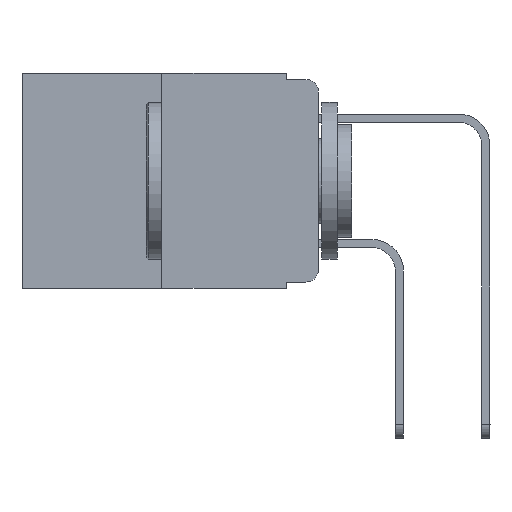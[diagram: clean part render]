
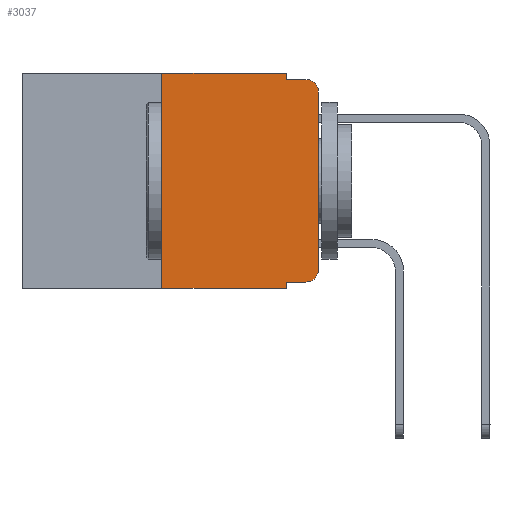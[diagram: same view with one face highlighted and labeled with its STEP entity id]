
A CAD part, left-side view. The second image highlights one B-rep face of the part: STEP entity #3037.
In plain terms, the highlighted planar face has unit normal (-1, 0, 0).
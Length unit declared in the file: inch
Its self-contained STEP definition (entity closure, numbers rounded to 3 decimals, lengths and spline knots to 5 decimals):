
#169 = EDGE_CURVE ( 'NONE', #7126, #14997, #2130, .T. ) ;
#392 = CARTESIAN_POINT ( 'NONE',  ( 0., 0.02, -0.333 ) ) ;
#841 = PLANE ( 'NONE',  #9326 ) ;
#935 = DIRECTION ( 'NONE',  ( 0., 0., -1. ) ) ;
#967 = CARTESIAN_POINT ( 'NONE',  ( 0., 0.051, 0. ) ) ;
#1067 = DIRECTION ( 'NONE',  ( 0., 0., 1. ) ) ;
#1392 = CARTESIAN_POINT ( 'NONE',  ( 0., 0.051, -0.343 ) ) ;
#2130 = LINE ( 'NONE', #6580, #14622 ) ;
#2162 = LINE ( 'NONE', #3811, #18434 ) ;
#2195 = ORIENTED_EDGE ( 'NONE', *, *, #14631, .F. ) ;
#2296 = LINE ( 'NONE', #12321, #9744 ) ;
#2407 = ORIENTED_EDGE ( 'NONE', *, *, #11637, .T. ) ;
#2442 = EDGE_CURVE ( 'NONE', #14997, #15102, #2162, .T. ) ;
#3037 = ADVANCED_FACE ( 'NONE', ( #14137 ), #841, .F. ) ;
#3051 = DIRECTION ( 'NONE',  ( 0., -1., 0. ) ) ;
#3281 = DIRECTION ( 'NONE',  ( 0., -1., 0. ) ) ;
#3811 = CARTESIAN_POINT ( 'NONE',  ( 0., 0.051, -0.01 ) ) ;
#4151 = AXIS2_PLACEMENT_3D ( 'NONE', #17323, #5757, #12860 ) ;
#4877 = DIRECTION ( 'NONE',  ( -1., 0., 0. ) ) ;
#5098 = ORIENTED_EDGE ( 'NONE', *, *, #17485, .T. ) ;
#5145 = CARTESIAN_POINT ( 'NONE',  ( 0., 0.051, -0.333 ) ) ;
#5186 = ORIENTED_EDGE ( 'NONE', *, *, #2442, .F. ) ;
#5389 = ORIENTED_EDGE ( 'NONE', *, *, #169, .F. ) ;
#5433 = CARTESIAN_POINT ( 'NONE',  ( 0., 0.25, 0. ) ) ;
#5496 = LINE ( 'NONE', #18900, #17254 ) ;
#5757 = DIRECTION ( 'NONE',  ( -1., 0., 0. ) ) ;
#6539 = CARTESIAN_POINT ( 'NONE',  ( 0., 0., -0.313 ) ) ;
#6580 = CARTESIAN_POINT ( 'NONE',  ( 0., 0.051, 0. ) ) ;
#6644 = VECTOR ( 'NONE', #1067, 39.37008 ) ;
#7014 = CARTESIAN_POINT ( 'NONE',  ( 0., 0.051, 0. ) ) ;
#7126 = VERTEX_POINT ( 'NONE', #967 ) ;
#7837 = VECTOR ( 'NONE', #18998, 39.37008 ) ;
#8096 = EDGE_CURVE ( 'NONE', #17822, #15102, #15632, .T. ) ;
#8347 = CARTESIAN_POINT ( 'NONE',  ( 0., 0.051, -0.01 ) ) ;
#8400 = LINE ( 'NONE', #17349, #7837 ) ;
#8668 = EDGE_CURVE ( 'NONE', #8718, #14617, #13019, .T. ) ;
#8718 = VERTEX_POINT ( 'NONE', #11445 ) ;
#8753 = LINE ( 'NONE', #7014, #16103 ) ;
#9326 = AXIS2_PLACEMENT_3D ( 'NONE', #18614, #11210, #935 ) ;
#9388 = CIRCLE ( 'NONE', #4151, 0.02 ) ;
#9744 = VECTOR ( 'NONE', #3281, 39.37008 ) ;
#9900 = CARTESIAN_POINT ( 'NONE',  ( 0., 0.02, -0.01 ) ) ;
#10445 = ORIENTED_EDGE ( 'NONE', *, *, #17111, .T. ) ;
#10681 = CARTESIAN_POINT ( 'NONE',  ( 0., 0.02, -0.03 ) ) ;
#10742 = VERTEX_POINT ( 'NONE', #6539 ) ;
#11030 = EDGE_CURVE ( 'NONE', #14617, #7126, #16356, .T. ) ;
#11061 = ORIENTED_EDGE ( 'NONE', *, *, #8096, .T. ) ;
#11210 = DIRECTION ( 'NONE',  ( 1., 0., 0. ) ) ;
#11274 = ORIENTED_EDGE ( 'NONE', *, *, #11030, .F. ) ;
#11407 = DIRECTION ( 'NONE',  ( 0., 0., 1. ) ) ;
#11445 = CARTESIAN_POINT ( 'NONE',  ( 0., 0.25, -0.343 ) ) ;
#11637 = EDGE_CURVE ( 'NONE', #10742, #17822, #5496, .T. ) ;
#12321 = CARTESIAN_POINT ( 'NONE',  ( 0., 0.051, -0.333 ) ) ;
#12448 = VERTEX_POINT ( 'NONE', #5145 ) ;
#12860 = DIRECTION ( 'NONE',  ( 0., 0., -1. ) ) ;
#13019 = LINE ( 'NONE', #5433, #6644 ) ;
#14078 = DIRECTION ( 'NONE',  ( 0., 0., -1. ) ) ;
#14091 = CARTESIAN_POINT ( 'NONE',  ( 0., 0., -0.03 ) ) ;
#14137 = FACE_OUTER_BOUND ( 'NONE', #15180, .T. ) ;
#14617 = VERTEX_POINT ( 'NONE', #15943 ) ;
#14622 = VECTOR ( 'NONE', #14078, 39.37008 ) ;
#14631 = EDGE_CURVE ( 'NONE', #12448, #17645, #8753, .T. ) ;
#14792 = VECTOR ( 'NONE', #3051, 39.37008 ) ;
#14997 = VERTEX_POINT ( 'NONE', #8347 ) ;
#15102 = VERTEX_POINT ( 'NONE', #9900 ) ;
#15180 = EDGE_LOOP ( 'NONE', ( #2407, #11061, #5186, #5389, #11274, #17889, #10445, #2195, #18988, #5098 ) ) ;
#15632 = CIRCLE ( 'NONE', #18740, 0.02 ) ;
#15746 = DIRECTION ( 'NONE',  ( 0., -1., 0. ) ) ;
#15943 = CARTESIAN_POINT ( 'NONE',  ( 0., 0.25, 0. ) ) ;
#16103 = VECTOR ( 'NONE', #16235, 39.37008 ) ;
#16235 = DIRECTION ( 'NONE',  ( 0., 0., -1. ) ) ;
#16356 = LINE ( 'NONE', #17819, #14792 ) ;
#16629 = DIRECTION ( 'NONE',  ( 0., 0., -1. ) ) ;
#17111 = EDGE_CURVE ( 'NONE', #8718, #17645, #8400, .T. ) ;
#17254 = VECTOR ( 'NONE', #11407, 39.37008 ) ;
#17323 = CARTESIAN_POINT ( 'NONE',  ( 0., 0.02, -0.313 ) ) ;
#17349 = CARTESIAN_POINT ( 'NONE',  ( 0., 0.473, -0.343 ) ) ;
#17485 = EDGE_CURVE ( 'NONE', #17816, #10742, #9388, .T. ) ;
#17645 = VERTEX_POINT ( 'NONE', #1392 ) ;
#17816 = VERTEX_POINT ( 'NONE', #392 ) ;
#17819 = CARTESIAN_POINT ( 'NONE',  ( 0., 0.473, 0. ) ) ;
#17822 = VERTEX_POINT ( 'NONE', #14091 ) ;
#17889 = ORIENTED_EDGE ( 'NONE', *, *, #8668, .F. ) ;
#18288 = EDGE_CURVE ( 'NONE', #12448, #17816, #2296, .T. ) ;
#18434 = VECTOR ( 'NONE', #15746, 39.37008 ) ;
#18614 = CARTESIAN_POINT ( 'NONE',  ( 0., 0.473, 0. ) ) ;
#18740 = AXIS2_PLACEMENT_3D ( 'NONE', #10681, #4877, #16629 ) ;
#18900 = CARTESIAN_POINT ( 'NONE',  ( 0., 0., 0. ) ) ;
#18988 = ORIENTED_EDGE ( 'NONE', *, *, #18288, .T. ) ;
#18998 = DIRECTION ( 'NONE',  ( 0., -1., 0. ) ) ;
